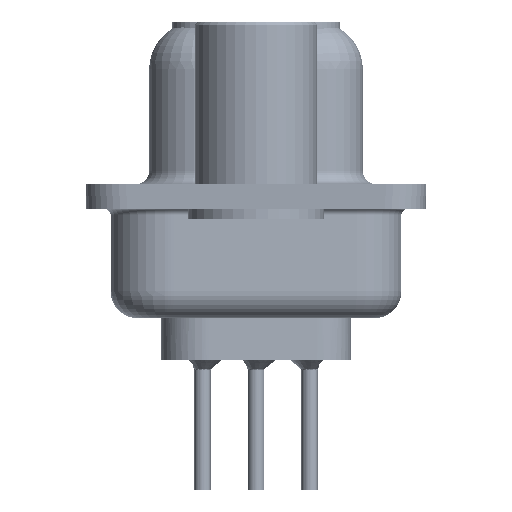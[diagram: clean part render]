
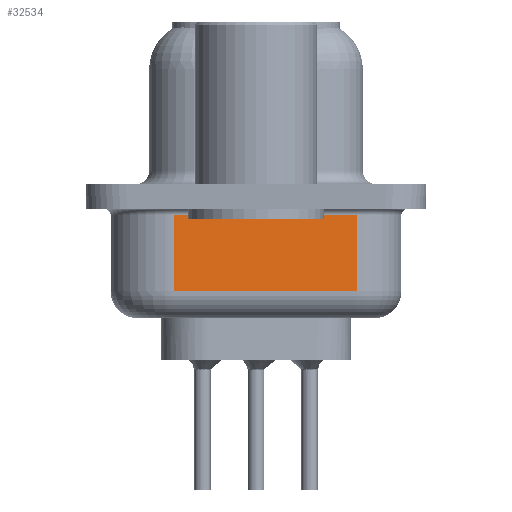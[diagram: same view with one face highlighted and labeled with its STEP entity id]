
A CAD part, left-side view. The second image highlights one B-rep face of the part: STEP entity #32534.
In plain terms, the highlighted planar face has unit normal (-0.985, -0.174, 0).
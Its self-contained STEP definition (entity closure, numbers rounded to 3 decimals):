
#1020 = CARTESIAN_POINT ( 'NONE',  ( 3., 3.028, -0.7 ) ) ;
#2471 = CARTESIAN_POINT ( 'NONE',  ( 4.191, -3.722, -3.5 ) ) ;
#3485 = VECTOR ( 'NONE', #36085, 1000. ) ;
#3554 = CARTESIAN_POINT ( 'NONE',  ( 3., 3.028, -4.5 ) ) ;
#4154 = EDGE_CURVE ( 'NONE', #29096, #12805, #6889, .T. ) ;
#4311 = LINE ( 'NONE', #1020, #3485 ) ;
#4831 = CARTESIAN_POINT ( 'NONE',  ( 4.191, -3.722, -4.5 ) ) ;
#5535 = VERTEX_POINT ( 'NONE', #18902 ) ;
#6889 = LINE ( 'NONE', #28767, #29007 ) ;
#8155 = LINE ( 'NONE', #4831, #19760 ) ;
#9012 = AXIS2_PLACEMENT_3D ( 'NONE', #13968, #39161, #27198 ) ;
#9936 = DIRECTION ( 'NONE',  ( 0., 0., 1. ) ) ;
#11564 = EDGE_CURVE ( 'NONE', #39007, #5535, #4311, .T. ) ;
#11813 = LINE ( 'NONE', #3554, #15015 ) ;
#12805 = VERTEX_POINT ( 'NONE', #2471 ) ;
#13316 = ORIENTED_EDGE ( 'NONE', *, *, #4154, .T. ) ;
#13968 = CARTESIAN_POINT ( 'NONE',  ( 3., 3.028, -4.5 ) ) ;
#14989 = ORIENTED_EDGE ( 'NONE', *, *, #34649, .F. ) ;
#15015 = VECTOR ( 'NONE', #9936, 1000. ) ;
#16000 = EDGE_LOOP ( 'NONE', ( #14989, #13316, #20349, #25462 ) ) ;
#18646 = DIRECTION ( 'NONE',  ( 0.174, -0.985, 0. ) ) ;
#18902 = CARTESIAN_POINT ( 'NONE',  ( 3., 3.028, -0.7 ) ) ;
#19457 = CARTESIAN_POINT ( 'NONE',  ( 3., 3.028, -3.5 ) ) ;
#19760 = VECTOR ( 'NONE', #27127, 1000. ) ;
#20349 = ORIENTED_EDGE ( 'NONE', *, *, #36577, .T. ) ;
#20799 = FACE_OUTER_BOUND ( 'NONE', #16000, .T. ) ;
#25462 = ORIENTED_EDGE ( 'NONE', *, *, #11564, .T. ) ;
#27127 = DIRECTION ( 'NONE',  ( 0., 0., 1. ) ) ;
#27198 = DIRECTION ( 'NONE',  ( -0.174, 0.985, 0. ) ) ;
#28767 = CARTESIAN_POINT ( 'NONE',  ( 3., 3.028, -3.5 ) ) ;
#29007 = VECTOR ( 'NONE', #18646, 1000. ) ;
#29096 = VERTEX_POINT ( 'NONE', #19457 ) ;
#32534 = ADVANCED_FACE ( 'NONE', ( #20799 ), #39366, .F. ) ;
#33587 = CARTESIAN_POINT ( 'NONE',  ( 4.191, -3.722, -0.7 ) ) ;
#34649 = EDGE_CURVE ( 'NONE', #29096, #5535, #11813, .T. ) ;
#36085 = DIRECTION ( 'NONE',  ( -0.174, 0.985, 0. ) ) ;
#36577 = EDGE_CURVE ( 'NONE', #12805, #39007, #8155, .T. ) ;
#39007 = VERTEX_POINT ( 'NONE', #33587 ) ;
#39161 = DIRECTION ( 'NONE',  ( 0.985, 0.174, 0. ) ) ;
#39366 = PLANE ( 'NONE',  #9012 ) ;
